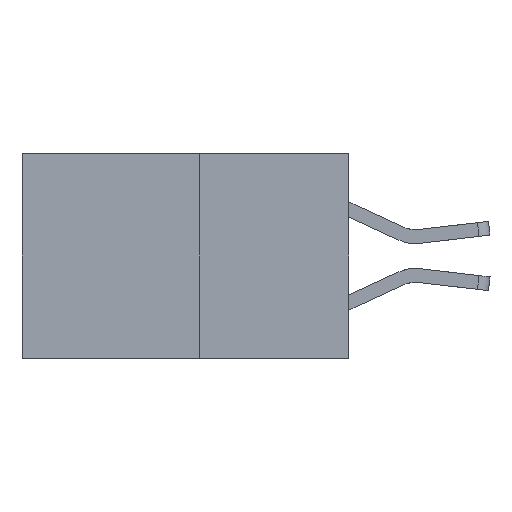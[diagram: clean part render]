
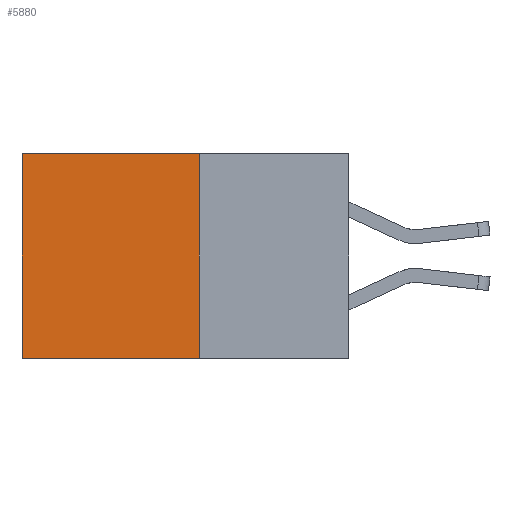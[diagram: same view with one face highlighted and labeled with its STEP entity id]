
A CAD part, left-side view. The second image highlights one B-rep face of the part: STEP entity #5880.
In plain terms, the highlighted planar face has unit normal (-1, 0, 0).
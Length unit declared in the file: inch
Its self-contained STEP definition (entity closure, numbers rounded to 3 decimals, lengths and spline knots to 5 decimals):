
#376 = AXIS2_PLACEMENT_3D ( 'NONE', #7022, #7047, #7106 ) ;
#1701 = CARTESIAN_POINT ( 'NONE',  ( 0.277, 0.59, -0.37 ) ) ;
#1851 = VERTEX_POINT ( 'NONE', #9545 ) ;
#1960 = LINE ( 'NONE', #6108, #6094 ) ;
#2371 = DIRECTION ( 'NONE',  ( 0., 1., 0. ) ) ;
#2788 = EDGE_CURVE ( 'NONE', #7790, #1851, #6786, .T. ) ;
#2805 = LINE ( 'NONE', #3090, #6880 ) ;
#2947 = EDGE_CURVE ( 'NONE', #1851, #7101, #4958, .T. ) ;
#3090 = CARTESIAN_POINT ( 'NONE',  ( 0.277, 0.27, -0.37 ) ) ;
#3456 = FACE_OUTER_BOUND ( 'NONE', #4995, .T. ) ;
#3913 = DIRECTION ( 'NONE',  ( 0., 0., -1. ) ) ;
#4356 = VECTOR ( 'NONE', #2371, 39.37008 ) ;
#4958 = LINE ( 'NONE', #7878, #10647 ) ;
#4995 = EDGE_LOOP ( 'NONE', ( #8798, #5526, #7857, #7800 ) ) ;
#5231 = CARTESIAN_POINT ( 'NONE',  ( 0.277, 0.27, 0. ) ) ;
#5360 = CARTESIAN_POINT ( 'NONE',  ( 0.277, 0.27, -0.37 ) ) ;
#5526 = ORIENTED_EDGE ( 'NONE', *, *, #8115, .F. ) ;
#5678 = VERTEX_POINT ( 'NONE', #5360 ) ;
#5880 = ADVANCED_FACE ( 'NONE', ( #3456 ), #6821, .F. ) ;
#6094 = VECTOR ( 'NONE', #6924, 39.37008 ) ;
#6108 = CARTESIAN_POINT ( 'NONE',  ( 0.277, 0.27, -0.37 ) ) ;
#6786 = LINE ( 'NONE', #5231, #4356 ) ;
#6821 = PLANE ( 'NONE',  #376 ) ;
#6880 = VECTOR ( 'NONE', #3913, 39.37008 ) ;
#6924 = DIRECTION ( 'NONE',  ( 0., 1., 0. ) ) ;
#7022 = CARTESIAN_POINT ( 'NONE',  ( 0.277, 0.27, -0.37 ) ) ;
#7047 = DIRECTION ( 'NONE',  ( 1., 0., 0. ) ) ;
#7101 = VERTEX_POINT ( 'NONE', #1701 ) ;
#7106 = DIRECTION ( 'NONE',  ( 0., 0., -1. ) ) ;
#7790 = VERTEX_POINT ( 'NONE', #8309 ) ;
#7800 = ORIENTED_EDGE ( 'NONE', *, *, #2788, .T. ) ;
#7847 = DIRECTION ( 'NONE',  ( 0., 0., -1. ) ) ;
#7857 = ORIENTED_EDGE ( 'NONE', *, *, #9307, .F. ) ;
#7878 = CARTESIAN_POINT ( 'NONE',  ( 0.277, 0.59, -0.37 ) ) ;
#8115 = EDGE_CURVE ( 'NONE', #5678, #7101, #1960, .T. ) ;
#8309 = CARTESIAN_POINT ( 'NONE',  ( 0.277, 0.27, 0. ) ) ;
#8798 = ORIENTED_EDGE ( 'NONE', *, *, #2947, .T. ) ;
#9307 = EDGE_CURVE ( 'NONE', #7790, #5678, #2805, .T. ) ;
#9545 = CARTESIAN_POINT ( 'NONE',  ( 0.277, 0.59, 0. ) ) ;
#10647 = VECTOR ( 'NONE', #7847, 39.37008 ) ;
